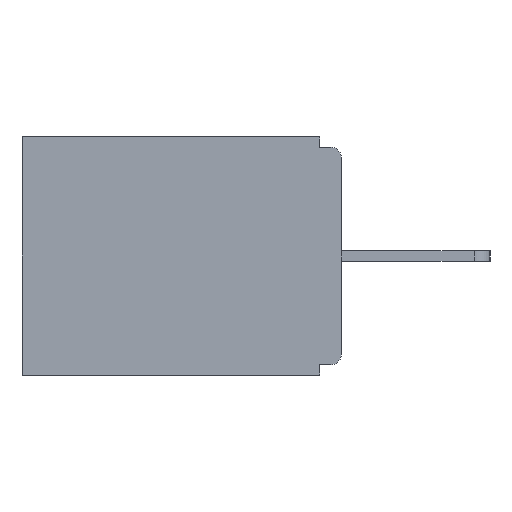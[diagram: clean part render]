
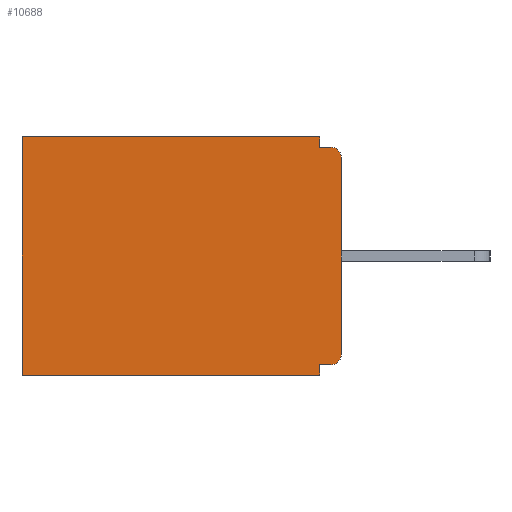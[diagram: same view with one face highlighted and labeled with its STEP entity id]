
A CAD part, left-side view. The second image highlights one B-rep face of the part: STEP entity #10688.
In plain terms, the highlighted planar face has unit normal (-1, 0, 0).
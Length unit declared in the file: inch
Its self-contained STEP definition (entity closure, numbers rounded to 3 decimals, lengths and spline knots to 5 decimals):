
#118 = CARTESIAN_POINT ( 'NONE',  ( 0.298, 0., -0.328 ) ) ;
#169 = EDGE_CURVE ( 'NONE', #2426, #3282, #9676, .T. ) ;
#377 = CIRCLE ( 'NONE', #2001, 0.015 ) ;
#384 = DIRECTION ( 'NONE',  ( -1., 0., 0. ) ) ;
#1335 = ORIENTED_EDGE ( 'NONE', *, *, #16253, .T. ) ;
#1402 = EDGE_CURVE ( 'NONE', #3282, #10355, #7590, .T. ) ;
#1537 = LINE ( 'NONE', #118, #12871 ) ;
#1667 = VECTOR ( 'NONE', #4304, 39.37008 ) ;
#1745 = VECTOR ( 'NONE', #5618, 39.37008 ) ;
#1853 = EDGE_LOOP ( 'NONE', ( #2997, #5344, #13882, #1335, #4647, #9521, #17923, #14443, #10689, #5195 ) ) ;
#2001 = AXIS2_PLACEMENT_3D ( 'NONE', #15549, #7061, #16926 ) ;
#2149 = VERTEX_POINT ( 'NONE', #4954 ) ;
#2243 = LINE ( 'NONE', #9035, #2744 ) ;
#2426 = VERTEX_POINT ( 'NONE', #7907 ) ;
#2581 = EDGE_CURVE ( 'NONE', #14782, #2149, #2243, .T. ) ;
#2744 = VECTOR ( 'NONE', #17110, 39.37008 ) ;
#2795 = VECTOR ( 'NONE', #7347, 39.37008 ) ;
#2804 = CARTESIAN_POINT ( 'NONE',  ( 0.298, 0., 0. ) ) ;
#2997 = ORIENTED_EDGE ( 'NONE', *, *, #16764, .T. ) ;
#3282 = VERTEX_POINT ( 'NONE', #14482 ) ;
#3300 = CARTESIAN_POINT ( 'NONE',  ( 0.298, 0., -0.343 ) ) ;
#4060 = CARTESIAN_POINT ( 'NONE',  ( 0.298, 0., -0.03 ) ) ;
#4125 = VERTEX_POINT ( 'NONE', #4349 ) ;
#4304 = DIRECTION ( 'NONE',  ( 0., 0., -1. ) ) ;
#4349 = CARTESIAN_POINT ( 'NONE',  ( 0.298, 0.46, 0. ) ) ;
#4647 = ORIENTED_EDGE ( 'NONE', *, *, #16215, .T. ) ;
#4954 = CARTESIAN_POINT ( 'NONE',  ( 0.298, 0.031, -0.015 ) ) ;
#5195 = ORIENTED_EDGE ( 'NONE', *, *, #10757, .F. ) ;
#5344 = ORIENTED_EDGE ( 'NONE', *, *, #17931, .F. ) ;
#5618 = DIRECTION ( 'NONE',  ( 0., -1., 0. ) ) ;
#5819 = CARTESIAN_POINT ( 'NONE',  ( 0.298, 0.46, 0. ) ) ;
#5903 = VECTOR ( 'NONE', #17262, 39.37008 ) ;
#6386 = LINE ( 'NONE', #2804, #5903 ) ;
#7061 = DIRECTION ( 'NONE',  ( -1., 0., 0. ) ) ;
#7347 = DIRECTION ( 'NONE',  ( 0., 0., -1. ) ) ;
#7590 = LINE ( 'NONE', #3300, #14670 ) ;
#7627 = VERTEX_POINT ( 'NONE', #4060 ) ;
#7717 = LINE ( 'NONE', #13193, #14796 ) ;
#7907 = CARTESIAN_POINT ( 'NONE',  ( 0.298, 0.031, -0.328 ) ) ;
#8730 = CARTESIAN_POINT ( 'NONE',  ( 0.298, 0., 0. ) ) ;
#8792 = PLANE ( 'NONE',  #18354 ) ;
#9035 = CARTESIAN_POINT ( 'NONE',  ( 0.298, 0.031, -0.343 ) ) ;
#9218 = CARTESIAN_POINT ( 'NONE',  ( 0.298, 0.015, -0.328 ) ) ;
#9410 = CARTESIAN_POINT ( 'NONE',  ( 0.298, 0.015, -0.313 ) ) ;
#9521 = ORIENTED_EDGE ( 'NONE', *, *, #1402, .F. ) ;
#9542 = EDGE_CURVE ( 'NONE', #14566, #2426, #1537, .T. ) ;
#9676 = LINE ( 'NONE', #16868, #1667 ) ;
#10232 = DIRECTION ( 'NONE',  ( 0., 0., -1. ) ) ;
#10355 = VERTEX_POINT ( 'NONE', #12241 ) ;
#10688 = ADVANCED_FACE ( 'NONE', ( #16093 ), #8792, .F. ) ;
#10689 = ORIENTED_EDGE ( 'NONE', *, *, #14611, .T. ) ;
#10690 = LINE ( 'NONE', #5819, #2795 ) ;
#10757 = EDGE_CURVE ( 'NONE', #7627, #12202, #7717, .T. ) ;
#10830 = DIRECTION ( 'NONE',  ( 0., 0., -1. ) ) ;
#10932 = VERTEX_POINT ( 'NONE', #12224 ) ;
#11190 = CARTESIAN_POINT ( 'NONE',  ( 0.298, 0.031, 0. ) ) ;
#11406 = DIRECTION ( 'NONE',  ( 0., 1., 0. ) ) ;
#12202 = VERTEX_POINT ( 'NONE', #16473 ) ;
#12224 = CARTESIAN_POINT ( 'NONE',  ( 0.298, 0.015, -0.015 ) ) ;
#12241 = CARTESIAN_POINT ( 'NONE',  ( 0.298, 0.46, -0.343 ) ) ;
#12871 = VECTOR ( 'NONE', #11406, 39.37008 ) ;
#13193 = CARTESIAN_POINT ( 'NONE',  ( 0.298, 0., 0. ) ) ;
#13882 = ORIENTED_EDGE ( 'NONE', *, *, #2581, .F. ) ;
#14443 = ORIENTED_EDGE ( 'NONE', *, *, #9542, .F. ) ;
#14482 = CARTESIAN_POINT ( 'NONE',  ( 0.298, 0.031, -0.343 ) ) ;
#14566 = VERTEX_POINT ( 'NONE', #9218 ) ;
#14585 = DIRECTION ( 'NONE',  ( 0., 0., -1. ) ) ;
#14611 = EDGE_CURVE ( 'NONE', #14566, #12202, #15948, .T. ) ;
#14670 = VECTOR ( 'NONE', #17359, 39.37008 ) ;
#14782 = VERTEX_POINT ( 'NONE', #11190 ) ;
#14796 = VECTOR ( 'NONE', #14585, 39.37008 ) ;
#15549 = CARTESIAN_POINT ( 'NONE',  ( 0.298, 0.015, -0.03 ) ) ;
#15686 = CARTESIAN_POINT ( 'NONE',  ( 0.298, 0., -0.015 ) ) ;
#15948 = CIRCLE ( 'NONE', #17852, 0.015 ) ;
#16093 = FACE_OUTER_BOUND ( 'NONE', #1853, .T. ) ;
#16215 = EDGE_CURVE ( 'NONE', #4125, #10355, #10690, .T. ) ;
#16253 = EDGE_CURVE ( 'NONE', #14782, #4125, #6386, .T. ) ;
#16473 = CARTESIAN_POINT ( 'NONE',  ( 0.298, 0., -0.313 ) ) ;
#16728 = LINE ( 'NONE', #15686, #1745 ) ;
#16764 = EDGE_CURVE ( 'NONE', #7627, #10932, #377, .T. ) ;
#16868 = CARTESIAN_POINT ( 'NONE',  ( 0.298, 0.031, -0.343 ) ) ;
#16926 = DIRECTION ( 'NONE',  ( 0., 0., -1. ) ) ;
#17110 = DIRECTION ( 'NONE',  ( 0., 0., -1. ) ) ;
#17262 = DIRECTION ( 'NONE',  ( 0., 1., 0. ) ) ;
#17359 = DIRECTION ( 'NONE',  ( 0., 1., 0. ) ) ;
#17852 = AXIS2_PLACEMENT_3D ( 'NONE', #9410, #384, #10830 ) ;
#17923 = ORIENTED_EDGE ( 'NONE', *, *, #169, .F. ) ;
#17931 = EDGE_CURVE ( 'NONE', #2149, #10932, #16728, .T. ) ;
#18354 = AXIS2_PLACEMENT_3D ( 'NONE', #8730, #18553, #10232 ) ;
#18553 = DIRECTION ( 'NONE',  ( 1., 0., 0. ) ) ;
